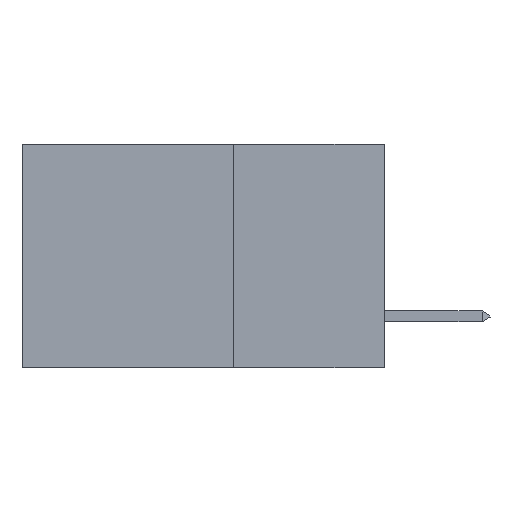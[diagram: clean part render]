
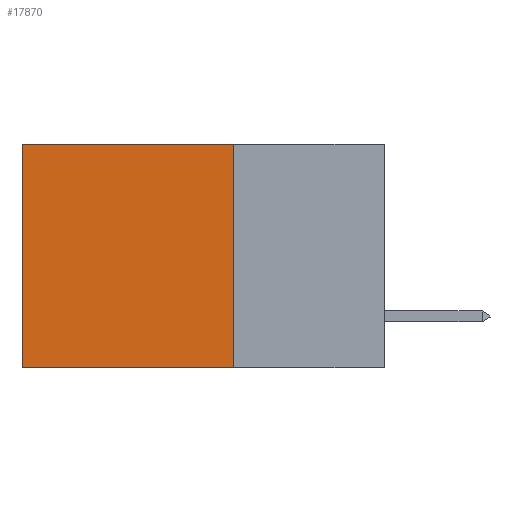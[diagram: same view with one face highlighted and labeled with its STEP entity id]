
A CAD part, left-side view. The second image highlights one B-rep face of the part: STEP entity #17870.
In plain terms, the highlighted planar face has unit normal (-1, 0, 0).
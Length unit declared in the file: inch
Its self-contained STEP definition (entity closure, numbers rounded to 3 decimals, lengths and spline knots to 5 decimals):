
#38 = VECTOR ( 'NONE', #20734, 39.37008 ) ;
#512 = EDGE_CURVE ( 'NONE', #26449, #38993, #44622, .T. ) ;
#1054 = DIRECTION ( 'NONE',  ( 0., 0., -1. ) ) ;
#1369 = LINE ( 'NONE', #28070, #19451 ) ;
#3658 = EDGE_CURVE ( 'NONE', #22589, #38993, #31134, .T. ) ;
#4600 = CARTESIAN_POINT ( 'NONE',  ( 0.2875, 0.25, 0. ) ) ;
#4969 = AXIS2_PLACEMENT_3D ( 'NONE', #14511, #36272, #1054 ) ;
#5791 = VECTOR ( 'NONE', #28029, 39.37008 ) ;
#9359 = EDGE_LOOP ( 'NONE', ( #33863, #38863, #19699, #14117 ) ) ;
#11944 = DIRECTION ( 'NONE',  ( 0., 1., 0. ) ) ;
#12139 = CARTESIAN_POINT ( 'NONE',  ( 0.2875, 0.6, -0.37 ) ) ;
#12355 = EDGE_CURVE ( 'NONE', #35041, #26449, #1369, .T. ) ;
#14117 = ORIENTED_EDGE ( 'NONE', *, *, #12355, .T. ) ;
#14511 = CARTESIAN_POINT ( 'NONE',  ( 0.2875, 0.25, 0. ) ) ;
#17870 = ADVANCED_FACE ( 'NONE', ( #17921 ), #41233, .F. ) ;
#17921 = FACE_OUTER_BOUND ( 'NONE', #9359, .T. ) ;
#19451 = VECTOR ( 'NONE', #11944, 39.37008 ) ;
#19699 = ORIENTED_EDGE ( 'NONE', *, *, #24204, .F. ) ;
#20734 = DIRECTION ( 'NONE',  ( 0., 0., -1. ) ) ;
#21191 = CARTESIAN_POINT ( 'NONE',  ( 0.2875, 0.25, -0.37 ) ) ;
#22589 = VERTEX_POINT ( 'NONE', #33454 ) ;
#23270 = CARTESIAN_POINT ( 'NONE',  ( 0.2875, 0.6, 0. ) ) ;
#24040 = CARTESIAN_POINT ( 'NONE',  ( 0.2875, 0.6, 0. ) ) ;
#24204 = EDGE_CURVE ( 'NONE', #35041, #22589, #40523, .T. ) ;
#25024 = VECTOR ( 'NONE', #31362, 39.37008 ) ;
#26449 = VERTEX_POINT ( 'NONE', #23270 ) ;
#28029 = DIRECTION ( 'NONE',  ( 0., 0., -1. ) ) ;
#28070 = CARTESIAN_POINT ( 'NONE',  ( 0.2875, 0.25, 0. ) ) ;
#31134 = LINE ( 'NONE', #21191, #25024 ) ;
#31362 = DIRECTION ( 'NONE',  ( 0., 1., 0. ) ) ;
#33454 = CARTESIAN_POINT ( 'NONE',  ( 0.2875, 0.25, -0.37 ) ) ;
#33863 = ORIENTED_EDGE ( 'NONE', *, *, #512, .T. ) ;
#35041 = VERTEX_POINT ( 'NONE', #4600 ) ;
#36272 = DIRECTION ( 'NONE',  ( 1., 0., 0. ) ) ;
#38863 = ORIENTED_EDGE ( 'NONE', *, *, #3658, .F. ) ;
#38993 = VERTEX_POINT ( 'NONE', #12139 ) ;
#40523 = LINE ( 'NONE', #44211, #38 ) ;
#41233 = PLANE ( 'NONE',  #4969 ) ;
#44211 = CARTESIAN_POINT ( 'NONE',  ( 0.2875, 0.25, 0. ) ) ;
#44622 = LINE ( 'NONE', #24040, #5791 ) ;
